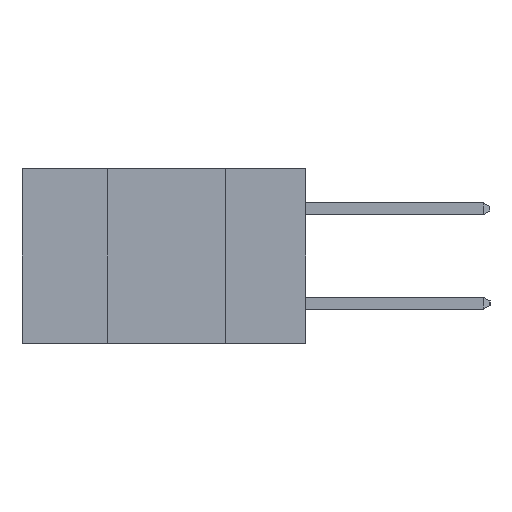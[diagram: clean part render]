
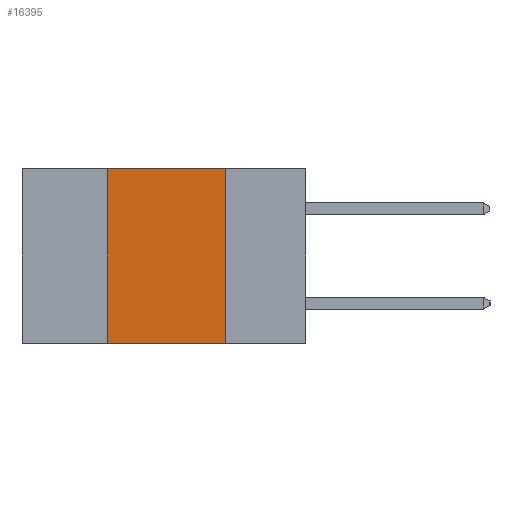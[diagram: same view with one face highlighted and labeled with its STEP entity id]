
A CAD part, left-side view. The second image highlights one B-rep face of the part: STEP entity #16395.
In plain terms, the highlighted planar face has unit normal (-1, 0, 0).
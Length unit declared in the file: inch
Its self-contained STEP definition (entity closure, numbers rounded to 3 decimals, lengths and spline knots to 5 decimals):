
#490 = VECTOR ( 'NONE', #10649, 39.37008 ) ;
#544 = LINE ( 'NONE', #13852, #10908 ) ;
#937 = LINE ( 'NONE', #17374, #490 ) ;
#2348 = DIRECTION ( 'NONE',  ( 1., 0., 0. ) ) ;
#5205 = EDGE_LOOP ( 'NONE', ( #9022, #6013, #13692, #11570 ) ) ;
#5259 = VERTEX_POINT ( 'NONE', #17465 ) ;
#6013 = ORIENTED_EDGE ( 'NONE', *, *, #17401, .F. ) ;
#6269 = VECTOR ( 'NONE', #13961, 39.37008 ) ;
#6971 = VERTEX_POINT ( 'NONE', #17691 ) ;
#7202 = FACE_OUTER_BOUND ( 'NONE', #5205, .T. ) ;
#7513 = CARTESIAN_POINT ( 'NONE',  ( 0., 0.17, -0.37 ) ) ;
#8021 = PLANE ( 'NONE',  #15610 ) ;
#9022 = ORIENTED_EDGE ( 'NONE', *, *, #16512, .F. ) ;
#10649 = DIRECTION ( 'NONE',  ( 0., 0., 1. ) ) ;
#10770 = CARTESIAN_POINT ( 'NONE',  ( 0., 0.6, 0. ) ) ;
#10908 = VECTOR ( 'NONE', #16550, 39.37008 ) ;
#11570 = ORIENTED_EDGE ( 'NONE', *, *, #11769, .T. ) ;
#11769 = EDGE_CURVE ( 'NONE', #6971, #15329, #544, .T. ) ;
#11913 = VECTOR ( 'NONE', #15111, 39.37008 ) ;
#12138 = DIRECTION ( 'NONE',  ( 0., 0., -1. ) ) ;
#12366 = CARTESIAN_POINT ( 'NONE',  ( 0., 0.17, -0.37 ) ) ;
#12592 = CARTESIAN_POINT ( 'NONE',  ( 0., 0.6, 0. ) ) ;
#12782 = LINE ( 'NONE', #12366, #11913 ) ;
#13692 = ORIENTED_EDGE ( 'NONE', *, *, #16322, .F. ) ;
#13852 = CARTESIAN_POINT ( 'NONE',  ( 0., 0.6, -0.37 ) ) ;
#13961 = DIRECTION ( 'NONE',  ( 0., -1., 0. ) ) ;
#14996 = VERTEX_POINT ( 'NONE', #16374 ) ;
#15111 = DIRECTION ( 'NONE',  ( 0., 0., -1. ) ) ;
#15329 = VERTEX_POINT ( 'NONE', #7513 ) ;
#15610 = AXIS2_PLACEMENT_3D ( 'NONE', #10770, #2348, #12138 ) ;
#16322 = EDGE_CURVE ( 'NONE', #6971, #14996, #937, .T. ) ;
#16374 = CARTESIAN_POINT ( 'NONE',  ( 0., 0.42, 0. ) ) ;
#16395 = ADVANCED_FACE ( 'NONE', ( #7202 ), #8021, .F. ) ;
#16512 = EDGE_CURVE ( 'NONE', #5259, #15329, #12782, .T. ) ;
#16550 = DIRECTION ( 'NONE',  ( 0., -1., 0. ) ) ;
#17139 = LINE ( 'NONE', #12592, #6269 ) ;
#17374 = CARTESIAN_POINT ( 'NONE',  ( 0., 0.42, -0.37 ) ) ;
#17401 = EDGE_CURVE ( 'NONE', #14996, #5259, #17139, .T. ) ;
#17465 = CARTESIAN_POINT ( 'NONE',  ( 0., 0.17, 0. ) ) ;
#17691 = CARTESIAN_POINT ( 'NONE',  ( 0., 0.42, -0.37 ) ) ;
